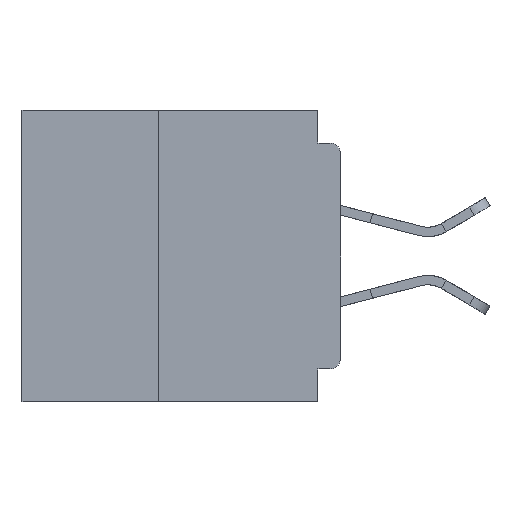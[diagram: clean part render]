
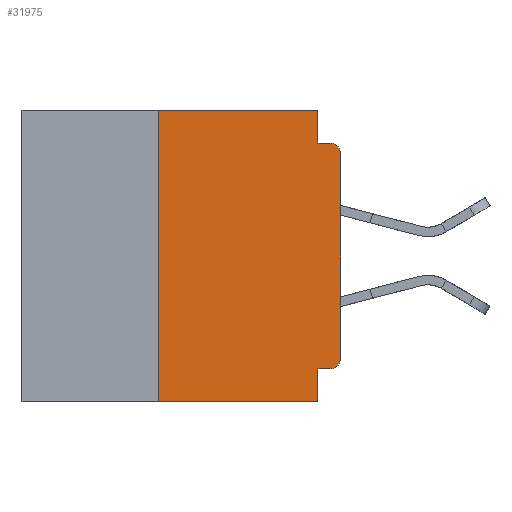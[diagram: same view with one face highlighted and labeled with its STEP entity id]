
A CAD part, left-side view. The second image highlights one B-rep face of the part: STEP entity #31975.
In plain terms, the highlighted planar face has unit normal (-1, 0, 0).
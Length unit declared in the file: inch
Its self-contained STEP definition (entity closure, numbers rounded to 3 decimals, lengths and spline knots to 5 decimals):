
#1041 = ORIENTED_EDGE ( 'NONE', *, *, #20361, .T. ) ;
#1347 = VERTEX_POINT ( 'NONE', #26881 ) ;
#2587 = VERTEX_POINT ( 'NONE', #3584 ) ;
#3275 = EDGE_CURVE ( 'NONE', #2587, #1347, #30142, .T. ) ;
#3340 = VECTOR ( 'NONE', #42655, 39.37008 ) ;
#3584 = CARTESIAN_POINT ( 'NONE',  ( 0., 0., -0.06 ) ) ;
#4132 = ORIENTED_EDGE ( 'NONE', *, *, #13557, .F. ) ;
#4402 = DIRECTION ( 'NONE',  ( 0., 0., 1. ) ) ;
#4495 = VECTOR ( 'NONE', #30965, 39.37008 ) ;
#4696 = VECTOR ( 'NONE', #44269, 39.37008 ) ;
#5388 = VECTOR ( 'NONE', #16779, 39.37008 ) ;
#7452 = VERTEX_POINT ( 'NONE', #19447 ) ;
#7522 = ORIENTED_EDGE ( 'NONE', *, *, #17648, .F. ) ;
#8103 = CARTESIAN_POINT ( 'NONE',  ( 0., 0.25, 0. ) ) ;
#8460 = PLANE ( 'NONE',  #26178 ) ;
#9130 = ORIENTED_EDGE ( 'NONE', *, *, #12175, .F. ) ;
#9297 = DIRECTION ( 'NONE',  ( 0., -1., 0. ) ) ;
#11119 = CARTESIAN_POINT ( 'NONE',  ( 0., 0.031, 0. ) ) ;
#11272 = CARTESIAN_POINT ( 'NONE',  ( 0., 0.25, -0.4 ) ) ;
#11576 = EDGE_CURVE ( 'NONE', #7452, #2587, #21952, .T. ) ;
#11845 = CARTESIAN_POINT ( 'NONE',  ( 0., 0.015, -0.34 ) ) ;
#12175 = EDGE_CURVE ( 'NONE', #48933, #30546, #45452, .T. ) ;
#12376 = CARTESIAN_POINT ( 'NONE',  ( 0., 0.437, 0. ) ) ;
#13339 = ORIENTED_EDGE ( 'NONE', *, *, #40288, .F. ) ;
#13557 = EDGE_CURVE ( 'NONE', #39042, #34743, #35745, .T. ) ;
#13773 = LINE ( 'NONE', #27077, #3340 ) ;
#14739 = AXIS2_PLACEMENT_3D ( 'NONE', #41167, #17961, #45031 ) ;
#15786 = DIRECTION ( 'NONE',  ( 0., 0., -1. ) ) ;
#16167 = CARTESIAN_POINT ( 'NONE',  ( 0., 0.015, -0.355 ) ) ;
#16319 = DIRECTION ( 'NONE',  ( 1., 0., 0. ) ) ;
#16734 = FACE_OUTER_BOUND ( 'NONE', #24724, .T. ) ;
#16779 = DIRECTION ( 'NONE',  ( 0., -1., 0. ) ) ;
#17163 = CARTESIAN_POINT ( 'NONE',  ( 0., 0.437, -0.4 ) ) ;
#17648 = EDGE_CURVE ( 'NONE', #19056, #1347, #22089, .T. ) ;
#17961 = DIRECTION ( 'NONE',  ( -1., 0., 0. ) ) ;
#19056 = VERTEX_POINT ( 'NONE', #43021 ) ;
#19447 = CARTESIAN_POINT ( 'NONE',  ( 0., 0., -0.34 ) ) ;
#20361 = EDGE_CURVE ( 'NONE', #39042, #7452, #50195, .T. ) ;
#20935 = CARTESIAN_POINT ( 'NONE',  ( 0., 0., -0.355 ) ) ;
#21017 = DIRECTION ( 'NONE',  ( 0., -1., 0. ) ) ;
#21611 = AXIS2_PLACEMENT_3D ( 'NONE', #11845, #39033, #15786 ) ;
#21952 = LINE ( 'NONE', #43161, #30989 ) ;
#22089 = LINE ( 'NONE', #24877, #43897 ) ;
#22653 = EDGE_CURVE ( 'NONE', #34041, #48933, #35547, .T. ) ;
#24585 = CARTESIAN_POINT ( 'NONE',  ( 0., 0.437, 0. ) ) ;
#24724 = EDGE_LOOP ( 'NONE', ( #42186, #49842, #7522, #13339, #9130, #40170, #30000, #48767, #4132, #1041 ) ) ;
#24877 = CARTESIAN_POINT ( 'NONE',  ( 0., 0., -0.045 ) ) ;
#26178 = AXIS2_PLACEMENT_3D ( 'NONE', #12376, #16319, #43427 ) ;
#26881 = CARTESIAN_POINT ( 'NONE',  ( 0., 0.015, -0.045 ) ) ;
#27077 = CARTESIAN_POINT ( 'NONE',  ( 0., 0.031, 0. ) ) ;
#28191 = CARTESIAN_POINT ( 'NONE',  ( 0., 0.031, -0.4 ) ) ;
#29170 = VECTOR ( 'NONE', #39181, 39.37008 ) ;
#30000 = ORIENTED_EDGE ( 'NONE', *, *, #32793, .T. ) ;
#30142 = CIRCLE ( 'NONE', #14739, 0.015 ) ;
#30546 = VERTEX_POINT ( 'NONE', #11119 ) ;
#30965 = DIRECTION ( 'NONE',  ( 0., 0., 1. ) ) ;
#30989 = VECTOR ( 'NONE', #4402, 39.37008 ) ;
#31157 = VERTEX_POINT ( 'NONE', #28191 ) ;
#31975 = ADVANCED_FACE ( 'NONE', ( #16734 ), #8460, .F. ) ;
#32793 = EDGE_CURVE ( 'NONE', #34041, #31157, #40918, .T. ) ;
#34041 = VERTEX_POINT ( 'NONE', #37229 ) ;
#34743 = VERTEX_POINT ( 'NONE', #45228 ) ;
#35090 = CARTESIAN_POINT ( 'NONE',  ( 0., 0.031, -0.4 ) ) ;
#35547 = LINE ( 'NONE', #11272, #4495 ) ;
#35745 = LINE ( 'NONE', #20935, #4696 ) ;
#37229 = CARTESIAN_POINT ( 'NONE',  ( 0., 0.25, -0.4 ) ) ;
#37767 = EDGE_CURVE ( 'NONE', #34743, #31157, #49706, .T. ) ;
#39033 = DIRECTION ( 'NONE',  ( -1., 0., 0. ) ) ;
#39042 = VERTEX_POINT ( 'NONE', #16167 ) ;
#39181 = DIRECTION ( 'NONE',  ( 0., 0., -1. ) ) ;
#40170 = ORIENTED_EDGE ( 'NONE', *, *, #22653, .F. ) ;
#40288 = EDGE_CURVE ( 'NONE', #30546, #19056, #13773, .T. ) ;
#40918 = LINE ( 'NONE', #17163, #47523 ) ;
#41167 = CARTESIAN_POINT ( 'NONE',  ( 0., 0.015, -0.06 ) ) ;
#42186 = ORIENTED_EDGE ( 'NONE', *, *, #11576, .T. ) ;
#42655 = DIRECTION ( 'NONE',  ( 0., 0., -1. ) ) ;
#43021 = CARTESIAN_POINT ( 'NONE',  ( 0., 0.031, -0.045 ) ) ;
#43161 = CARTESIAN_POINT ( 'NONE',  ( 0., 0., 0. ) ) ;
#43427 = DIRECTION ( 'NONE',  ( 0., 0., -1. ) ) ;
#43897 = VECTOR ( 'NONE', #21017, 39.37008 ) ;
#44269 = DIRECTION ( 'NONE',  ( 0., 1., 0. ) ) ;
#45031 = DIRECTION ( 'NONE',  ( 0., 0., -1. ) ) ;
#45228 = CARTESIAN_POINT ( 'NONE',  ( 0., 0.031, -0.355 ) ) ;
#45452 = LINE ( 'NONE', #24585, #5388 ) ;
#47523 = VECTOR ( 'NONE', #9297, 39.37008 ) ;
#48767 = ORIENTED_EDGE ( 'NONE', *, *, #37767, .F. ) ;
#48933 = VERTEX_POINT ( 'NONE', #8103 ) ;
#49706 = LINE ( 'NONE', #35090, #29170 ) ;
#49842 = ORIENTED_EDGE ( 'NONE', *, *, #3275, .T. ) ;
#50195 = CIRCLE ( 'NONE', #21611, 0.015 ) ;
